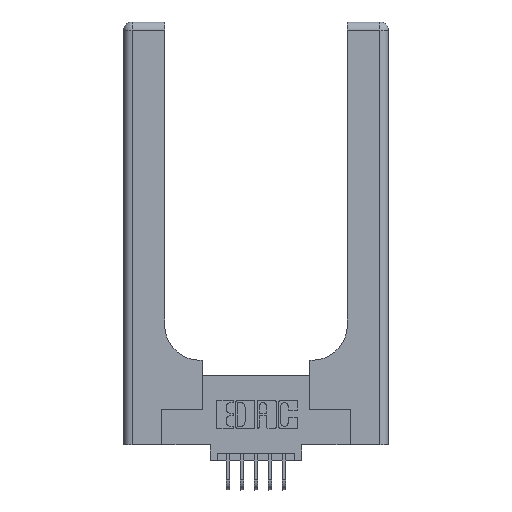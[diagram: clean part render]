
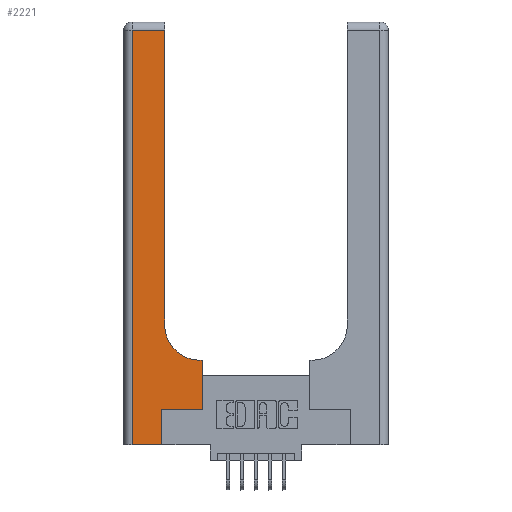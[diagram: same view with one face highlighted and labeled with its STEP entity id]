
A CAD part, top view. The second image highlights one B-rep face of the part: STEP entity #2221.
In plain terms, the highlighted planar face has unit normal (0, 0, 1).
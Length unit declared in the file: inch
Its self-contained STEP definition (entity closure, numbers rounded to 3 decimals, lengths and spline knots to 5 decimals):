
#373 = VECTOR ( 'NONE', #13445, 39.37008 ) ;
#424 = CARTESIAN_POINT ( 'NONE',  ( 0.269, 0., 0.37 ) ) ;
#565 = EDGE_CURVE ( 'NONE', #5896, #10638, #1219, .T. ) ;
#707 = EDGE_CURVE ( 'NONE', #10638, #14962, #3135, .T. ) ;
#1081 = CARTESIAN_POINT ( 'NONE',  ( 0., 3., 0.37 ) ) ;
#1191 = DIRECTION ( 'NONE',  ( -1., 0., 0. ) ) ;
#1219 = LINE ( 'NONE', #10463, #10045 ) ;
#1602 = EDGE_LOOP ( 'NONE', ( #4478, #8446, #13748, #12156, #11465, #11111, #6049, #9817, #10039 ) ) ;
#1777 = CARTESIAN_POINT ( 'NONE',  ( 0.5585, 0.25, 0.37 ) ) ;
#2049 = EDGE_CURVE ( 'NONE', #11431, #4161, #5598, .T. ) ;
#2112 = CARTESIAN_POINT ( 'NONE',  ( 0.06, 0., 0.37 ) ) ;
#2221 = ADVANCED_FACE ( 'NONE', ( #12474 ), #7366, .F. ) ;
#2284 = EDGE_CURVE ( 'NONE', #4161, #5896, #5776, .T. ) ;
#2382 = DIRECTION ( 'NONE',  ( 0., 0., -1. ) ) ;
#3135 = LINE ( 'NONE', #3143, #10985 ) ;
#3143 = CARTESIAN_POINT ( 'NONE',  ( 0.2915, 0.6, 0.37 ) ) ;
#3556 = DIRECTION ( 'NONE',  ( 0., 1., 0. ) ) ;
#3682 = VECTOR ( 'NONE', #11307, 39.37008 ) ;
#4161 = VERTEX_POINT ( 'NONE', #7085 ) ;
#4287 = CARTESIAN_POINT ( 'NONE',  ( 0.5415, 0.85, 0.37 ) ) ;
#4478 = ORIENTED_EDGE ( 'NONE', *, *, #15272, .T. ) ;
#5401 = VECTOR ( 'NONE', #13222, 39.37008 ) ;
#5487 = AXIS2_PLACEMENT_3D ( 'NONE', #1081, #2382, #1191 ) ;
#5568 = CARTESIAN_POINT ( 'NONE',  ( 0.5415, 0.6, 0.37 ) ) ;
#5598 = LINE ( 'NONE', #424, #3682 ) ;
#5714 = CARTESIAN_POINT ( 'NONE',  ( 0., 2.94, 0.37 ) ) ;
#5776 = LINE ( 'NONE', #13452, #5401 ) ;
#5896 = VERTEX_POINT ( 'NONE', #1777 ) ;
#6049 = ORIENTED_EDGE ( 'NONE', *, *, #565, .T. ) ;
#6161 = VERTEX_POINT ( 'NONE', #13297 ) ;
#6191 = VERTEX_POINT ( 'NONE', #10198 ) ;
#6775 = LINE ( 'NONE', #15104, #14048 ) ;
#7085 = CARTESIAN_POINT ( 'NONE',  ( 0.269, 0.25, 0.37 ) ) ;
#7187 = VECTOR ( 'NONE', #10619, 39.37008 ) ;
#7366 = PLANE ( 'NONE',  #5487 ) ;
#7675 = LINE ( 'NONE', #7971, #14950 ) ;
#7971 = CARTESIAN_POINT ( 'NONE',  ( 0.2915, 3., 0.37 ) ) ;
#8043 = DIRECTION ( 'NONE',  ( 1., 0., 0. ) ) ;
#8446 = ORIENTED_EDGE ( 'NONE', *, *, #11692, .T. ) ;
#8927 = CARTESIAN_POINT ( 'NONE',  ( 0.06, 2.94, 0.37 ) ) ;
#9018 = DIRECTION ( 'NONE',  ( 0., -1., 0. ) ) ;
#9540 = EDGE_CURVE ( 'NONE', #14962, #6161, #11310, .T. ) ;
#9817 = ORIENTED_EDGE ( 'NONE', *, *, #707, .T. ) ;
#10039 = ORIENTED_EDGE ( 'NONE', *, *, #9540, .T. ) ;
#10045 = VECTOR ( 'NONE', #3556, 39.37008 ) ;
#10149 = CARTESIAN_POINT ( 'NONE',  ( 0.269, 0., 0.37 ) ) ;
#10198 = CARTESIAN_POINT ( 'NONE',  ( 0.2915, 2.94, 0.37 ) ) ;
#10463 = CARTESIAN_POINT ( 'NONE',  ( 0.5585, 0.25, 0.37 ) ) ;
#10577 = DIRECTION ( 'NONE',  ( -1., 0., 0. ) ) ;
#10619 = DIRECTION ( 'NONE',  ( -1., 0., 0. ) ) ;
#10638 = VERTEX_POINT ( 'NONE', #15436 ) ;
#10980 = CARTESIAN_POINT ( 'NONE',  ( 0., 0., 0.37 ) ) ;
#10985 = VECTOR ( 'NONE', #10577, 39.37008 ) ;
#11111 = ORIENTED_EDGE ( 'NONE', *, *, #2284, .T. ) ;
#11307 = DIRECTION ( 'NONE',  ( 0., 1., 0. ) ) ;
#11310 = CIRCLE ( 'NONE', #13647, 0.25 ) ;
#11431 = VERTEX_POINT ( 'NONE', #10149 ) ;
#11465 = ORIENTED_EDGE ( 'NONE', *, *, #2049, .T. ) ;
#11692 = EDGE_CURVE ( 'NONE', #6191, #15875, #13697, .T. ) ;
#11773 = VERTEX_POINT ( 'NONE', #2112 ) ;
#12156 = ORIENTED_EDGE ( 'NONE', *, *, #15043, .T. ) ;
#12474 = FACE_OUTER_BOUND ( 'NONE', #1602, .T. ) ;
#12704 = EDGE_CURVE ( 'NONE', #15875, #11773, #6775, .T. ) ;
#13222 = DIRECTION ( 'NONE',  ( 1., 0., 0. ) ) ;
#13297 = CARTESIAN_POINT ( 'NONE',  ( 0.2915, 0.85, 0.37 ) ) ;
#13445 = DIRECTION ( 'NONE',  ( 1., 0., 0. ) ) ;
#13452 = CARTESIAN_POINT ( 'NONE',  ( 0.269, 0.25, 0.37 ) ) ;
#13595 = LINE ( 'NONE', #10980, #373 ) ;
#13647 = AXIS2_PLACEMENT_3D ( 'NONE', #4287, #14066, #8043 ) ;
#13697 = LINE ( 'NONE', #5714, #7187 ) ;
#13748 = ORIENTED_EDGE ( 'NONE', *, *, #12704, .T. ) ;
#14048 = VECTOR ( 'NONE', #9018, 39.37008 ) ;
#14066 = DIRECTION ( 'NONE',  ( 0., 0., -1. ) ) ;
#14950 = VECTOR ( 'NONE', #15453, 39.37008 ) ;
#14962 = VERTEX_POINT ( 'NONE', #5568 ) ;
#15043 = EDGE_CURVE ( 'NONE', #11773, #11431, #13595, .T. ) ;
#15104 = CARTESIAN_POINT ( 'NONE',  ( 0.06, 3., 0.37 ) ) ;
#15272 = EDGE_CURVE ( 'NONE', #6161, #6191, #7675, .T. ) ;
#15436 = CARTESIAN_POINT ( 'NONE',  ( 0.5585, 0.6, 0.37 ) ) ;
#15453 = DIRECTION ( 'NONE',  ( 0., 1., 0. ) ) ;
#15875 = VERTEX_POINT ( 'NONE', #8927 ) ;
